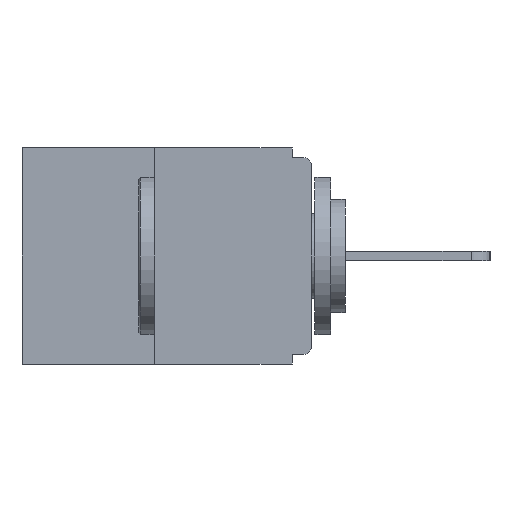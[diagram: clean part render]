
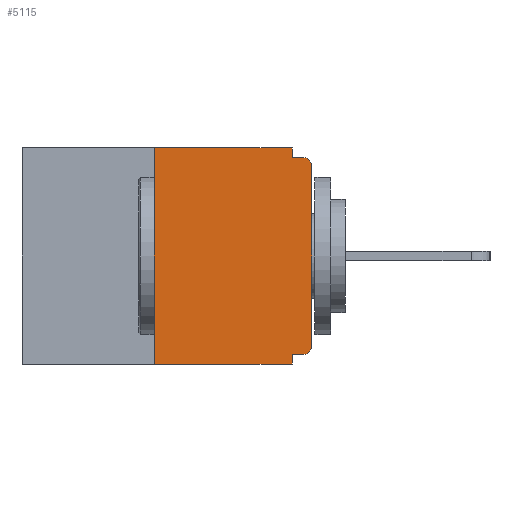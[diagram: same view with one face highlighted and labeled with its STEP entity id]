
A CAD part, left-side view. The second image highlights one B-rep face of the part: STEP entity #5115.
In plain terms, the highlighted planar face has unit normal (-1, 0, 0).
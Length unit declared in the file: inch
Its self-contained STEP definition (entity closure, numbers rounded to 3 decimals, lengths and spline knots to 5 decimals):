
#81 = VERTEX_POINT ( 'NONE', #6528 ) ;
#133 = VERTEX_POINT ( 'NONE', #3324 ) ;
#258 = VERTEX_POINT ( 'NONE', #12859 ) ;
#298 = EDGE_CURVE ( 'NONE', #81, #133, #4681, .T. ) ;
#532 = DIRECTION ( 'NONE',  ( 0., -1., 0. ) ) ;
#543 = ORIENTED_EDGE ( 'NONE', *, *, #1935, .F. ) ;
#558 = EDGE_CURVE ( 'NONE', #6570, #81, #11065, .T. ) ;
#981 = CARTESIAN_POINT ( 'NONE',  ( 0., 0.031, 0. ) ) ;
#1034 = EDGE_CURVE ( 'NONE', #133, #258, #10037, .T. ) ;
#1038 = VERTEX_POINT ( 'NONE', #6242 ) ;
#1507 = VECTOR ( 'NONE', #10990, 39.37008 ) ;
#1551 = EDGE_CURVE ( 'NONE', #6570, #10151, #12072, .T. ) ;
#1588 = DIRECTION ( 'NONE',  ( 0., 0., -1. ) ) ;
#1935 = EDGE_CURVE ( 'NONE', #1038, #3398, #13835, .T. ) ;
#2132 = EDGE_CURVE ( 'NONE', #1038, #7530, #8651, .T. ) ;
#2238 = CARTESIAN_POINT ( 'NONE',  ( 0., 0.46, 0. ) ) ;
#2332 = EDGE_CURVE ( 'NONE', #10151, #7530, #14689, .T. ) ;
#2438 = EDGE_CURVE ( 'NONE', #9313, #7818, #13544, .T. ) ;
#2738 = VECTOR ( 'NONE', #532, 39.37008 ) ;
#3185 = CARTESIAN_POINT ( 'NONE',  ( 0., 0.031, 0. ) ) ;
#3324 = CARTESIAN_POINT ( 'NONE',  ( 0., 0., -0.03 ) ) ;
#3398 = VERTEX_POINT ( 'NONE', #3752 ) ;
#3554 = DIRECTION ( 'NONE',  ( 0., 0., -1. ) ) ;
#3752 = CARTESIAN_POINT ( 'NONE',  ( 0., 0.25, 0. ) ) ;
#4038 = DIRECTION ( 'NONE',  ( 0., -1., 0. ) ) ;
#4372 = ORIENTED_EDGE ( 'NONE', *, *, #2132, .T. ) ;
#4681 = LINE ( 'NONE', #6919, #10528 ) ;
#4721 = EDGE_CURVE ( 'NONE', #3398, #9313, #14489, .T. ) ;
#4810 = DIRECTION ( 'NONE',  ( 0., 0., -1. ) ) ;
#5115 = ADVANCED_FACE ( 'NONE', ( #9597 ), #9507, .F. ) ;
#5371 = DIRECTION ( 'NONE',  ( -1., 0., 0. ) ) ;
#5404 = VECTOR ( 'NONE', #5583, 39.37008 ) ;
#5583 = DIRECTION ( 'NONE',  ( 0., -1., 0. ) ) ;
#5959 = EDGE_CURVE ( 'NONE', #7818, #258, #9167, .T. ) ;
#6179 = VECTOR ( 'NONE', #12719, 39.37008 ) ;
#6242 = CARTESIAN_POINT ( 'NONE',  ( 0., 0.25, -0.343 ) ) ;
#6349 = EDGE_LOOP ( 'NONE', ( #12954, #543, #4372, #6415, #6709, #6747, #6761, #6855, #7010, #7117 ) ) ;
#6415 = ORIENTED_EDGE ( 'NONE', *, *, #2332, .F. ) ;
#6528 = CARTESIAN_POINT ( 'NONE',  ( 0., 0., -0.313 ) ) ;
#6570 = VERTEX_POINT ( 'NONE', #8158 ) ;
#6709 = ORIENTED_EDGE ( 'NONE', *, *, #1551, .F. ) ;
#6732 = AXIS2_PLACEMENT_3D ( 'NONE', #14674, #5371, #1588 ) ;
#6747 = ORIENTED_EDGE ( 'NONE', *, *, #558, .T. ) ;
#6759 = CARTESIAN_POINT ( 'NONE',  ( 0., 0.031, -0.343 ) ) ;
#6761 = ORIENTED_EDGE ( 'NONE', *, *, #298, .T. ) ;
#6855 = ORIENTED_EDGE ( 'NONE', *, *, #1034, .T. ) ;
#6919 = CARTESIAN_POINT ( 'NONE',  ( 0., 0., 0. ) ) ;
#7010 = ORIENTED_EDGE ( 'NONE', *, *, #5959, .F. ) ;
#7117 = ORIENTED_EDGE ( 'NONE', *, *, #2438, .F. ) ;
#7504 = CARTESIAN_POINT ( 'NONE',  ( 0., 0.031, -0.015 ) ) ;
#7530 = VERTEX_POINT ( 'NONE', #6759 ) ;
#7818 = VERTEX_POINT ( 'NONE', #7504 ) ;
#7836 = DIRECTION ( 'NONE',  ( 0., 0., 1. ) ) ;
#8158 = CARTESIAN_POINT ( 'NONE',  ( 0., 0.015, -0.328 ) ) ;
#8651 = LINE ( 'NONE', #11347, #5404 ) ;
#9167 = LINE ( 'NONE', #14137, #2738 ) ;
#9313 = VERTEX_POINT ( 'NONE', #981 ) ;
#9507 = PLANE ( 'NONE',  #12319 ) ;
#9523 = VECTOR ( 'NONE', #4810, 39.37008 ) ;
#9597 = FACE_OUTER_BOUND ( 'NONE', #6349, .T. ) ;
#9875 = CARTESIAN_POINT ( 'NONE',  ( 0., 0.015, -0.313 ) ) ;
#10037 = CIRCLE ( 'NONE', #6732, 0.015 ) ;
#10074 = DIRECTION ( 'NONE',  ( -1., 0., 0. ) ) ;
#10151 = VERTEX_POINT ( 'NONE', #11726 ) ;
#10239 = CARTESIAN_POINT ( 'NONE',  ( 0., 0.031, -0.343 ) ) ;
#10528 = VECTOR ( 'NONE', #7836, 39.37008 ) ;
#10566 = DIRECTION ( 'NONE',  ( 1., 0., 0. ) ) ;
#10643 = CARTESIAN_POINT ( 'NONE',  ( 0., 0., -0.328 ) ) ;
#10873 = CARTESIAN_POINT ( 'NONE',  ( 0., 0.25, 0. ) ) ;
#10990 = DIRECTION ( 'NONE',  ( 0., 0., -1. ) ) ;
#11065 = CIRCLE ( 'NONE', #12843, 0.015 ) ;
#11347 = CARTESIAN_POINT ( 'NONE',  ( 0., 0.46, -0.343 ) ) ;
#11726 = CARTESIAN_POINT ( 'NONE',  ( 0., 0.031, -0.328 ) ) ;
#11888 = DIRECTION ( 'NONE',  ( 0., 0., -1. ) ) ;
#11970 = CARTESIAN_POINT ( 'NONE',  ( 0., 0.46, 0. ) ) ;
#12072 = LINE ( 'NONE', #10643, #6179 ) ;
#12319 = AXIS2_PLACEMENT_3D ( 'NONE', #2238, #10566, #3554 ) ;
#12719 = DIRECTION ( 'NONE',  ( 0., 1., 0. ) ) ;
#12843 = AXIS2_PLACEMENT_3D ( 'NONE', #9875, #10074, #11888 ) ;
#12859 = CARTESIAN_POINT ( 'NONE',  ( 0., 0.015, -0.015 ) ) ;
#12954 = ORIENTED_EDGE ( 'NONE', *, *, #4721, .F. ) ;
#13017 = DIRECTION ( 'NONE',  ( 0., 0., 1. ) ) ;
#13544 = LINE ( 'NONE', #3185, #1507 ) ;
#13553 = VECTOR ( 'NONE', #13017, 39.37008 ) ;
#13835 = LINE ( 'NONE', #10873, #13553 ) ;
#14137 = CARTESIAN_POINT ( 'NONE',  ( 0., 0., -0.015 ) ) ;
#14189 = VECTOR ( 'NONE', #4038, 39.37008 ) ;
#14489 = LINE ( 'NONE', #11970, #14189 ) ;
#14674 = CARTESIAN_POINT ( 'NONE',  ( 0., 0.015, -0.03 ) ) ;
#14689 = LINE ( 'NONE', #10239, #9523 ) ;
